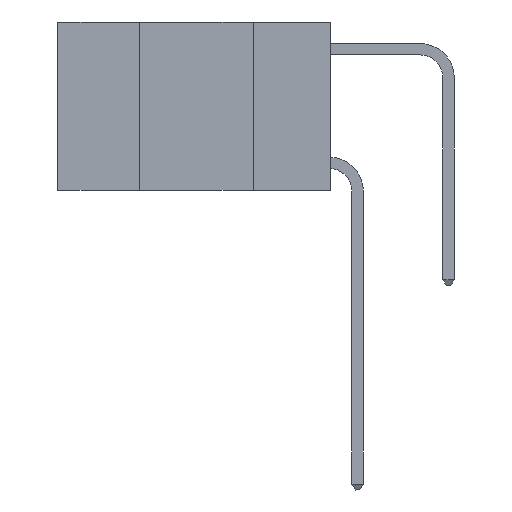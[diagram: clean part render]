
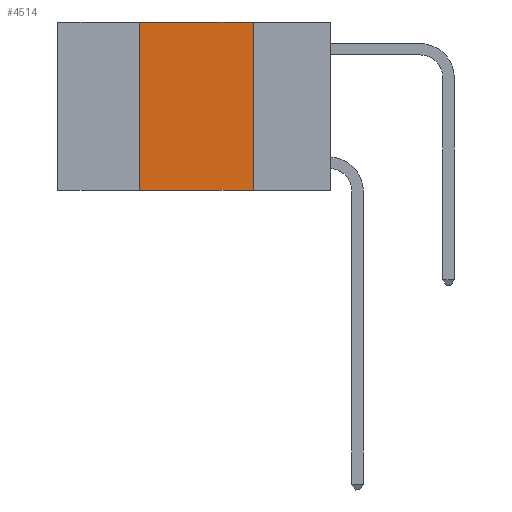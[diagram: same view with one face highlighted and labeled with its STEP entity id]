
A CAD part, left-side view. The second image highlights one B-rep face of the part: STEP entity #4514.
In plain terms, the highlighted planar face has unit normal (-1, 0, 0).
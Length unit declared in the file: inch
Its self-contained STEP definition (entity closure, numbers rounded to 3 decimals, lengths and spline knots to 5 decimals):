
#125 = ORIENTED_EDGE ( 'NONE', *, *, #5970, .F. ) ;
#571 = AXIS2_PLACEMENT_3D ( 'NONE', #10224, #4737, #11113 ) ;
#706 = VECTOR ( 'NONE', #10837, 39.37008 ) ;
#749 = FACE_OUTER_BOUND ( 'NONE', #1971, .T. ) ;
#922 = VERTEX_POINT ( 'NONE', #7021 ) ;
#1516 = VERTEX_POINT ( 'NONE', #8965 ) ;
#1971 = EDGE_LOOP ( 'NONE', ( #125, #5068, #10951, #6219 ) ) ;
#2030 = PLANE ( 'NONE',  #571 ) ;
#3277 = CARTESIAN_POINT ( 'NONE',  ( 0., 0.17, 0. ) ) ;
#3463 = VERTEX_POINT ( 'NONE', #10363 ) ;
#3617 = VECTOR ( 'NONE', #8109, 39.37008 ) ;
#3897 = LINE ( 'NONE', #5283, #3617 ) ;
#4233 = VERTEX_POINT ( 'NONE', #3277 ) ;
#4471 = CARTESIAN_POINT ( 'NONE',  ( 0., 0.42, 0. ) ) ;
#4503 = CARTESIAN_POINT ( 'NONE',  ( 0., 0.6, -0.37 ) ) ;
#4514 = ADVANCED_FACE ( 'NONE', ( #749 ), #2030, .F. ) ;
#4531 = VECTOR ( 'NONE', #9600, 39.37008 ) ;
#4737 = DIRECTION ( 'NONE',  ( 1., 0., 0. ) ) ;
#4819 = LINE ( 'NONE', #8700, #4531 ) ;
#5068 = ORIENTED_EDGE ( 'NONE', *, *, #8753, .F. ) ;
#5173 = LINE ( 'NONE', #4503, #10055 ) ;
#5283 = CARTESIAN_POINT ( 'NONE',  ( 0., 0.17, 0. ) ) ;
#5970 = EDGE_CURVE ( 'NONE', #4233, #1516, #3897, .T. ) ;
#6006 = EDGE_CURVE ( 'NONE', #3463, #922, #7954, .T. ) ;
#6008 = EDGE_CURVE ( 'NONE', #3463, #1516, #5173, .T. ) ;
#6219 = ORIENTED_EDGE ( 'NONE', *, *, #6008, .T. ) ;
#7021 = CARTESIAN_POINT ( 'NONE',  ( 0., 0.42, 0. ) ) ;
#7954 = LINE ( 'NONE', #4471, #706 ) ;
#8109 = DIRECTION ( 'NONE',  ( 0., 0., -1. ) ) ;
#8700 = CARTESIAN_POINT ( 'NONE',  ( 0., 0.6, 0. ) ) ;
#8753 = EDGE_CURVE ( 'NONE', #922, #4233, #4819, .T. ) ;
#8965 = CARTESIAN_POINT ( 'NONE',  ( 0., 0.17, -0.37 ) ) ;
#9600 = DIRECTION ( 'NONE',  ( 0., -1., 0. ) ) ;
#10055 = VECTOR ( 'NONE', #10873, 39.37008 ) ;
#10224 = CARTESIAN_POINT ( 'NONE',  ( 0., 0.6, 0. ) ) ;
#10363 = CARTESIAN_POINT ( 'NONE',  ( 0., 0.42, -0.37 ) ) ;
#10837 = DIRECTION ( 'NONE',  ( 0., 0., 1. ) ) ;
#10873 = DIRECTION ( 'NONE',  ( 0., -1., 0. ) ) ;
#10951 = ORIENTED_EDGE ( 'NONE', *, *, #6006, .F. ) ;
#11113 = DIRECTION ( 'NONE',  ( 0., 0., -1. ) ) ;
